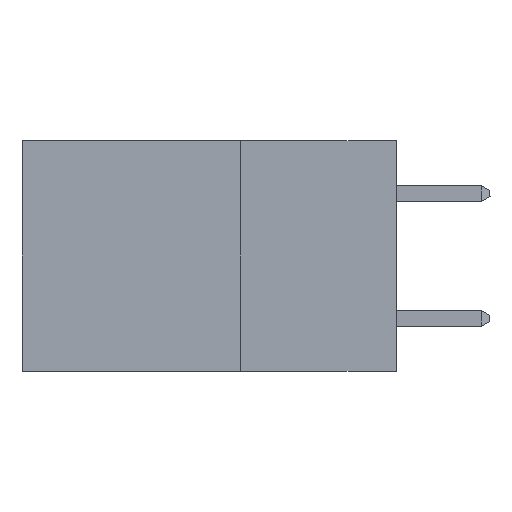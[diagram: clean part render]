
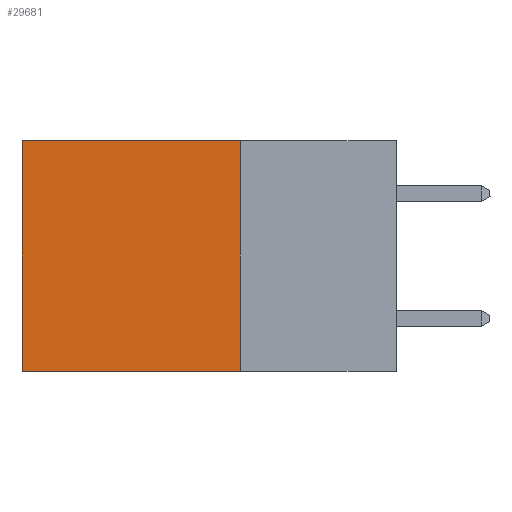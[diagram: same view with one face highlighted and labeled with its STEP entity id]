
A CAD part, left-side view. The second image highlights one B-rep face of the part: STEP entity #29681.
In plain terms, the highlighted planar face has unit normal (-1, 0, 0).
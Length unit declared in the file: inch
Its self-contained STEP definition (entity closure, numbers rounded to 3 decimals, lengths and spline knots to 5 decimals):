
#86 = VECTOR ( 'NONE', #23289, 39.37008 ) ;
#727 = ORIENTED_EDGE ( 'NONE', *, *, #29393, .T. ) ;
#967 = VERTEX_POINT ( 'NONE', #8151 ) ;
#2715 = EDGE_CURVE ( 'NONE', #10737, #7091, #13194, .T. ) ;
#3091 = VECTOR ( 'NONE', #27587, 39.37008 ) ;
#3317 = DIRECTION ( 'NONE',  ( 0., 0., -1. ) ) ;
#3766 = LINE ( 'NONE', #16512, #86 ) ;
#4535 = ORIENTED_EDGE ( 'NONE', *, *, #12488, .F. ) ;
#5085 = ORIENTED_EDGE ( 'NONE', *, *, #2715, .T. ) ;
#5890 = ORIENTED_EDGE ( 'NONE', *, *, #17105, .F. ) ;
#6782 = CARTESIAN_POINT ( 'NONE',  ( 0.298, 0.25, 0. ) ) ;
#7091 = VERTEX_POINT ( 'NONE', #20709 ) ;
#7921 = VECTOR ( 'NONE', #18324, 39.37008 ) ;
#8151 = CARTESIAN_POINT ( 'NONE',  ( 0.298, 0.25, 0. ) ) ;
#9382 = LINE ( 'NONE', #6782, #13318 ) ;
#9389 = CARTESIAN_POINT ( 'NONE',  ( 0.298, 0.6, 0. ) ) ;
#10038 = PLANE ( 'NONE',  #13206 ) ;
#10737 = VERTEX_POINT ( 'NONE', #9389 ) ;
#12348 = CARTESIAN_POINT ( 'NONE',  ( 0.298, 0.25, 0. ) ) ;
#12488 = EDGE_CURVE ( 'NONE', #25804, #7091, #20173, .T. ) ;
#13194 = LINE ( 'NONE', #25118, #3091 ) ;
#13206 = AXIS2_PLACEMENT_3D ( 'NONE', #12348, #28474, #14235 ) ;
#13318 = VECTOR ( 'NONE', #3317, 39.37008 ) ;
#13658 = CARTESIAN_POINT ( 'NONE',  ( 0.298, 0.25, -0.37 ) ) ;
#14235 = DIRECTION ( 'NONE',  ( 0., 0., -1. ) ) ;
#15958 = CARTESIAN_POINT ( 'NONE',  ( 0.298, 0.25, -0.37 ) ) ;
#16512 = CARTESIAN_POINT ( 'NONE',  ( 0.298, 0.25, 0. ) ) ;
#17105 = EDGE_CURVE ( 'NONE', #967, #25804, #9382, .T. ) ;
#18324 = DIRECTION ( 'NONE',  ( 0., 1., 0. ) ) ;
#20173 = LINE ( 'NONE', #15958, #7921 ) ;
#20709 = CARTESIAN_POINT ( 'NONE',  ( 0.298, 0.6, -0.37 ) ) ;
#22330 = EDGE_LOOP ( 'NONE', ( #5085, #4535, #5890, #727 ) ) ;
#23289 = DIRECTION ( 'NONE',  ( 0., 1., 0. ) ) ;
#25118 = CARTESIAN_POINT ( 'NONE',  ( 0.298, 0.6, 0. ) ) ;
#25804 = VERTEX_POINT ( 'NONE', #13658 ) ;
#27587 = DIRECTION ( 'NONE',  ( 0., 0., -1. ) ) ;
#27882 = FACE_OUTER_BOUND ( 'NONE', #22330, .T. ) ;
#28474 = DIRECTION ( 'NONE',  ( 1., 0., 0. ) ) ;
#29393 = EDGE_CURVE ( 'NONE', #967, #10737, #3766, .T. ) ;
#29681 = ADVANCED_FACE ( 'NONE', ( #27882 ), #10038, .F. ) ;
